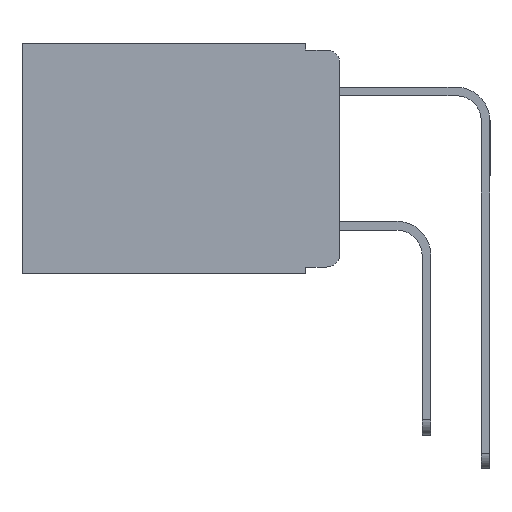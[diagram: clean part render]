
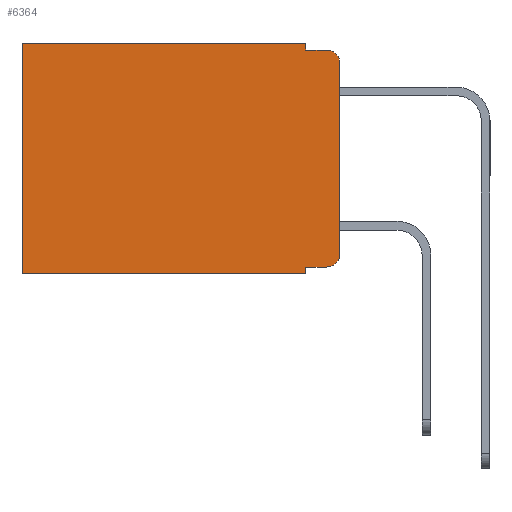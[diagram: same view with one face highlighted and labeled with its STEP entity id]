
A CAD part, left-side view. The second image highlights one B-rep face of the part: STEP entity #6364.
In plain terms, the highlighted planar face has unit normal (-1, 0, 0).
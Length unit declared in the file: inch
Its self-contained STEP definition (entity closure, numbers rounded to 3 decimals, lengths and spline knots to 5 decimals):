
#133 = AXIS2_PLACEMENT_3D ( 'NONE', #10201, #1650, #11584 ) ;
#299 = EDGE_CURVE ( 'NONE', #10996, #4191, #3407, .T. ) ;
#505 = ORIENTED_EDGE ( 'NONE', *, *, #516, .T. ) ;
#516 = EDGE_CURVE ( 'NONE', #1807, #5249, #10388, .T. ) ;
#517 = CARTESIAN_POINT ( 'NONE',  ( 0.298, 0.051, -0.343 ) ) ;
#866 = ORIENTED_EDGE ( 'NONE', *, *, #17383, .F. ) ;
#993 = VECTOR ( 'NONE', #2581, 39.37008 ) ;
#1069 = DIRECTION ( 'NONE',  ( 0., 0., -1. ) ) ;
#1158 = CARTESIAN_POINT ( 'NONE',  ( 0.298, 0.051, 0. ) ) ;
#1452 = CARTESIAN_POINT ( 'NONE',  ( 0.298, 0.051, 0. ) ) ;
#1650 = DIRECTION ( 'NONE',  ( -1., 0., 0. ) ) ;
#1668 = CARTESIAN_POINT ( 'NONE',  ( 0.298, 0., 0. ) ) ;
#1807 = VERTEX_POINT ( 'NONE', #1452 ) ;
#1895 = VERTEX_POINT ( 'NONE', #17778 ) ;
#2218 = CARTESIAN_POINT ( 'NONE',  ( 0.298, 0., -0.313 ) ) ;
#2281 = CARTESIAN_POINT ( 'NONE',  ( 0.298, 0.051, -0.333 ) ) ;
#2316 = ORIENTED_EDGE ( 'NONE', *, *, #9324, .F. ) ;
#2318 = VERTEX_POINT ( 'NONE', #3476 ) ;
#2347 = ORIENTED_EDGE ( 'NONE', *, *, #14135, .T. ) ;
#2498 = ORIENTED_EDGE ( 'NONE', *, *, #3589, .F. ) ;
#2581 = DIRECTION ( 'NONE',  ( 0., 0., -1. ) ) ;
#2788 = EDGE_CURVE ( 'NONE', #7800, #13747, #8514, .T. ) ;
#2794 = AXIS2_PLACEMENT_3D ( 'NONE', #1668, #14359, #5921 ) ;
#3197 = CARTESIAN_POINT ( 'NONE',  ( 0.298, 0.051, -0.333 ) ) ;
#3228 = ORIENTED_EDGE ( 'NONE', *, *, #299, .F. ) ;
#3372 = CARTESIAN_POINT ( 'NONE',  ( 0.298, 0., 0. ) ) ;
#3407 = LINE ( 'NONE', #10444, #10156 ) ;
#3451 = LINE ( 'NONE', #2281, #10206 ) ;
#3476 = CARTESIAN_POINT ( 'NONE',  ( 0.298, 0.02, -0.01 ) ) ;
#3491 = LINE ( 'NONE', #5636, #10256 ) ;
#3589 = EDGE_CURVE ( 'NONE', #1895, #13747, #3491, .T. ) ;
#4067 = DIRECTION ( 'NONE',  ( 0., 0., -1. ) ) ;
#4191 = VERTEX_POINT ( 'NONE', #16491 ) ;
#4707 = EDGE_LOOP ( 'NONE', ( #2498, #2347, #866, #7962, #505, #15435, #3228, #2316, #15621, #9912 ) ) ;
#4748 = LINE ( 'NONE', #1158, #993 ) ;
#5031 = LINE ( 'NONE', #11220, #8462 ) ;
#5249 = VERTEX_POINT ( 'NONE', #14676 ) ;
#5636 = CARTESIAN_POINT ( 'NONE',  ( 0.298, 0., 0. ) ) ;
#5921 = DIRECTION ( 'NONE',  ( 0., 0., -1. ) ) ;
#6364 = ADVANCED_FACE ( 'NONE', ( #6600 ), #12962, .F. ) ;
#6439 = DIRECTION ( 'NONE',  ( 0., 0., -1. ) ) ;
#6538 = VECTOR ( 'NONE', #10147, 39.37008 ) ;
#6600 = FACE_OUTER_BOUND ( 'NONE', #4707, .T. ) ;
#6626 = EDGE_CURVE ( 'NONE', #13051, #7800, #3451, .T. ) ;
#7008 = DIRECTION ( 'NONE',  ( 0., 1., 0. ) ) ;
#7800 = VERTEX_POINT ( 'NONE', #12211 ) ;
#7941 = EDGE_CURVE ( 'NONE', #1807, #9718, #4748, .T. ) ;
#7962 = ORIENTED_EDGE ( 'NONE', *, *, #7941, .F. ) ;
#8462 = VECTOR ( 'NONE', #4067, 39.37008 ) ;
#8514 = CIRCLE ( 'NONE', #17664, 0.02 ) ;
#8564 = LINE ( 'NONE', #9608, #15473 ) ;
#9324 = EDGE_CURVE ( 'NONE', #13051, #10996, #8564, .T. ) ;
#9608 = CARTESIAN_POINT ( 'NONE',  ( 0.298, 0.051, 0. ) ) ;
#9718 = VERTEX_POINT ( 'NONE', #16035 ) ;
#9912 = ORIENTED_EDGE ( 'NONE', *, *, #2788, .T. ) ;
#10147 = DIRECTION ( 'NONE',  ( 0., 1., 0. ) ) ;
#10156 = VECTOR ( 'NONE', #7008, 39.37008 ) ;
#10201 = CARTESIAN_POINT ( 'NONE',  ( 0.298, 0.02, -0.03 ) ) ;
#10206 = VECTOR ( 'NONE', #10819, 39.37008 ) ;
#10256 = VECTOR ( 'NONE', #1069, 39.37008 ) ;
#10334 = VECTOR ( 'NONE', #15037, 39.37008 ) ;
#10388 = LINE ( 'NONE', #3372, #6538 ) ;
#10444 = CARTESIAN_POINT ( 'NONE',  ( 0.298, 0., -0.343 ) ) ;
#10819 = DIRECTION ( 'NONE',  ( 0., -1., 0. ) ) ;
#10996 = VERTEX_POINT ( 'NONE', #517 ) ;
#11220 = CARTESIAN_POINT ( 'NONE',  ( 0.298, 0.473, 0. ) ) ;
#11584 = DIRECTION ( 'NONE',  ( 0., 0., -1. ) ) ;
#12144 = CARTESIAN_POINT ( 'NONE',  ( 0.298, 0.02, -0.313 ) ) ;
#12211 = CARTESIAN_POINT ( 'NONE',  ( 0.298, 0.02, -0.333 ) ) ;
#12416 = EDGE_CURVE ( 'NONE', #5249, #4191, #5031, .T. ) ;
#12962 = PLANE ( 'NONE',  #2794 ) ;
#13051 = VERTEX_POINT ( 'NONE', #3197 ) ;
#13655 = CARTESIAN_POINT ( 'NONE',  ( 0.298, 0.051, -0.01 ) ) ;
#13747 = VERTEX_POINT ( 'NONE', #2218 ) ;
#14135 = EDGE_CURVE ( 'NONE', #1895, #2318, #16185, .T. ) ;
#14359 = DIRECTION ( 'NONE',  ( 1., 0., 0. ) ) ;
#14676 = CARTESIAN_POINT ( 'NONE',  ( 0.298, 0.473, 0. ) ) ;
#15037 = DIRECTION ( 'NONE',  ( 0., -1., 0. ) ) ;
#15435 = ORIENTED_EDGE ( 'NONE', *, *, #12416, .T. ) ;
#15473 = VECTOR ( 'NONE', #17808, 39.37008 ) ;
#15621 = ORIENTED_EDGE ( 'NONE', *, *, #6626, .T. ) ;
#16035 = CARTESIAN_POINT ( 'NONE',  ( 0.298, 0.051, -0.01 ) ) ;
#16185 = CIRCLE ( 'NONE', #133, 0.02 ) ;
#16491 = CARTESIAN_POINT ( 'NONE',  ( 0.298, 0.473, -0.343 ) ) ;
#17187 = LINE ( 'NONE', #13655, #10334 ) ;
#17383 = EDGE_CURVE ( 'NONE', #9718, #2318, #17187, .T. ) ;
#17522 = DIRECTION ( 'NONE',  ( -1., 0., 0. ) ) ;
#17664 = AXIS2_PLACEMENT_3D ( 'NONE', #12144, #17522, #6439 ) ;
#17778 = CARTESIAN_POINT ( 'NONE',  ( 0.298, 0., -0.03 ) ) ;
#17808 = DIRECTION ( 'NONE',  ( 0., 0., -1. ) ) ;
